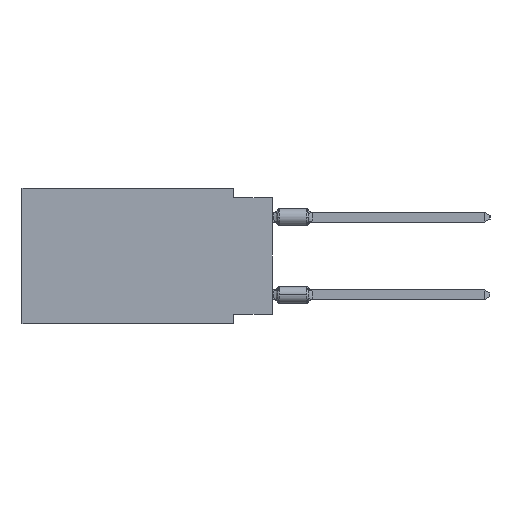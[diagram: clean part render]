
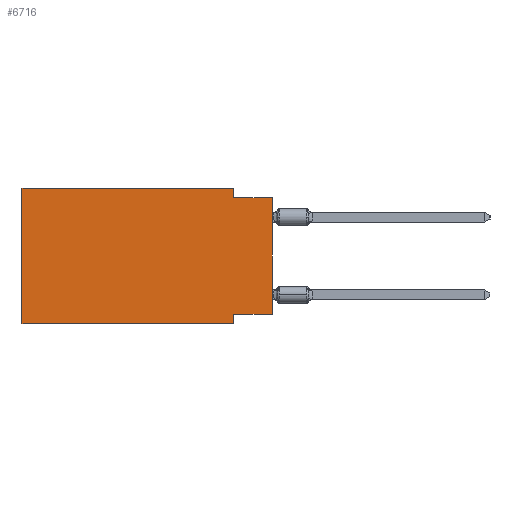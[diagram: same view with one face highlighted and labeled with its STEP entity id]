
A CAD part, left-side view. The second image highlights one B-rep face of the part: STEP entity #6716.
In plain terms, the highlighted planar face has unit normal (-1, 0, 0).
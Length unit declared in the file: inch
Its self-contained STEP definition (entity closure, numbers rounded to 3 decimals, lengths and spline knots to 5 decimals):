
#570 = CARTESIAN_POINT ( 'NONE',  ( 0., 0.645, 0. ) ) ;
#1813 = EDGE_CURVE ( 'NONE', #34738, #29547, #6159, .T. ) ;
#3307 = DIRECTION ( 'NONE',  ( 0., -1., 0. ) ) ;
#3727 = ORIENTED_EDGE ( 'NONE', *, *, #8596, .F. ) ;
#3745 = DIRECTION ( 'NONE',  ( 0., 0., -1. ) ) ;
#3969 = VECTOR ( 'NONE', #6434, 39.37008 ) ;
#4417 = VERTEX_POINT ( 'NONE', #21090 ) ;
#5248 = EDGE_CURVE ( 'NONE', #38832, #18186, #6274, .T. ) ;
#5866 = CARTESIAN_POINT ( 'NONE',  ( 0., 0.645, -0.35 ) ) ;
#6159 = LINE ( 'NONE', #20946, #8182 ) ;
#6274 = LINE ( 'NONE', #5866, #35825 ) ;
#6434 = DIRECTION ( 'NONE',  ( 0., -1., 0. ) ) ;
#6716 = ADVANCED_FACE ( 'NONE', ( #13765 ), #15594, .F. ) ;
#6961 = ORIENTED_EDGE ( 'NONE', *, *, #5248, .T. ) ;
#7676 = AXIS2_PLACEMENT_3D ( 'NONE', #570, #12642, #3745 ) ;
#8182 = VECTOR ( 'NONE', #27574, 39.37008 ) ;
#8596 = EDGE_CURVE ( 'NONE', #34738, #12036, #38861, .T. ) ;
#8695 = CARTESIAN_POINT ( 'NONE',  ( 0., 0., -0.325 ) ) ;
#8829 = CARTESIAN_POINT ( 'NONE',  ( 0., 0.1, 0. ) ) ;
#9168 = EDGE_CURVE ( 'NONE', #38832, #20641, #20331, .T. ) ;
#9220 = DIRECTION ( 'NONE',  ( 0., 1., 0. ) ) ;
#9450 = CARTESIAN_POINT ( 'NONE',  ( 0., 0.1, -0.025 ) ) ;
#9669 = EDGE_CURVE ( 'NONE', #20641, #4417, #13334, .T. ) ;
#10304 = EDGE_CURVE ( 'NONE', #13941, #29547, #35587, .T. ) ;
#10425 = ORIENTED_EDGE ( 'NONE', *, *, #18052, .F. ) ;
#10580 = CARTESIAN_POINT ( 'NONE',  ( 0., 0.645, 0. ) ) ;
#12036 = VERTEX_POINT ( 'NONE', #16496 ) ;
#12094 = ORIENTED_EDGE ( 'NONE', *, *, #10304, .F. ) ;
#12642 = DIRECTION ( 'NONE',  ( 1., 0., 0. ) ) ;
#13302 = VECTOR ( 'NONE', #30408, 39.37008 ) ;
#13334 = LINE ( 'NONE', #18654, #3969 ) ;
#13765 = FACE_OUTER_BOUND ( 'NONE', #34384, .T. ) ;
#13941 = VERTEX_POINT ( 'NONE', #9450 ) ;
#15410 = CARTESIAN_POINT ( 'NONE',  ( 0., 0.1, -0.35 ) ) ;
#15594 = PLANE ( 'NONE',  #7676 ) ;
#16496 = CARTESIAN_POINT ( 'NONE',  ( 0., 0.1, -0.325 ) ) ;
#16559 = ORIENTED_EDGE ( 'NONE', *, *, #9168, .F. ) ;
#17378 = CARTESIAN_POINT ( 'NONE',  ( 0., 0.645, 0. ) ) ;
#18052 = EDGE_CURVE ( 'NONE', #12036, #18186, #24040, .T. ) ;
#18186 = VERTEX_POINT ( 'NONE', #15410 ) ;
#18484 = LINE ( 'NONE', #8829, #13302 ) ;
#18654 = CARTESIAN_POINT ( 'NONE',  ( 0., 0.645, 0. ) ) ;
#20331 = LINE ( 'NONE', #17378, #22158 ) ;
#20641 = VERTEX_POINT ( 'NONE', #10580 ) ;
#20946 = CARTESIAN_POINT ( 'NONE',  ( 0., 0., 0. ) ) ;
#21090 = CARTESIAN_POINT ( 'NONE',  ( 0., 0.1, 0. ) ) ;
#22158 = VECTOR ( 'NONE', #32437, 39.37008 ) ;
#22774 = VECTOR ( 'NONE', #9220, 39.37008 ) ;
#23036 = VECTOR ( 'NONE', #29908, 39.37008 ) ;
#23056 = ORIENTED_EDGE ( 'NONE', *, *, #32332, .F. ) ;
#24040 = LINE ( 'NONE', #26966, #23036 ) ;
#25888 = CARTESIAN_POINT ( 'NONE',  ( 0., 0.645, -0.35 ) ) ;
#26966 = CARTESIAN_POINT ( 'NONE',  ( 0., 0.1, -0.35 ) ) ;
#27574 = DIRECTION ( 'NONE',  ( 0., 0., 1. ) ) ;
#29547 = VERTEX_POINT ( 'NONE', #37371 ) ;
#29722 = CARTESIAN_POINT ( 'NONE',  ( 0., 0., -0.025 ) ) ;
#29908 = DIRECTION ( 'NONE',  ( 0., 0., -1. ) ) ;
#30408 = DIRECTION ( 'NONE',  ( 0., 0., -1. ) ) ;
#32332 = EDGE_CURVE ( 'NONE', #4417, #13941, #18484, .T. ) ;
#32437 = DIRECTION ( 'NONE',  ( 0., 0., 1. ) ) ;
#32845 = DIRECTION ( 'NONE',  ( 0., -1., 0. ) ) ;
#33148 = CARTESIAN_POINT ( 'NONE',  ( 0., 0., -0.325 ) ) ;
#34094 = VECTOR ( 'NONE', #32845, 39.37008 ) ;
#34384 = EDGE_LOOP ( 'NONE', ( #34589, #12094, #23056, #36893, #16559, #6961, #10425, #3727 ) ) ;
#34589 = ORIENTED_EDGE ( 'NONE', *, *, #1813, .T. ) ;
#34738 = VERTEX_POINT ( 'NONE', #8695 ) ;
#35587 = LINE ( 'NONE', #29722, #34094 ) ;
#35825 = VECTOR ( 'NONE', #3307, 39.37008 ) ;
#36893 = ORIENTED_EDGE ( 'NONE', *, *, #9669, .F. ) ;
#37371 = CARTESIAN_POINT ( 'NONE',  ( 0., 0., -0.025 ) ) ;
#38832 = VERTEX_POINT ( 'NONE', #25888 ) ;
#38861 = LINE ( 'NONE', #33148, #22774 ) ;
